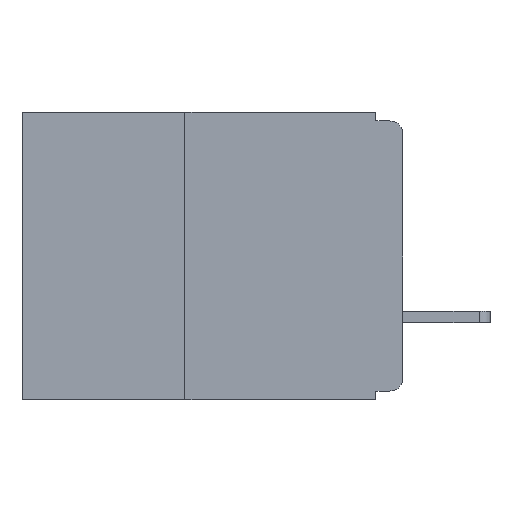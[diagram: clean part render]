
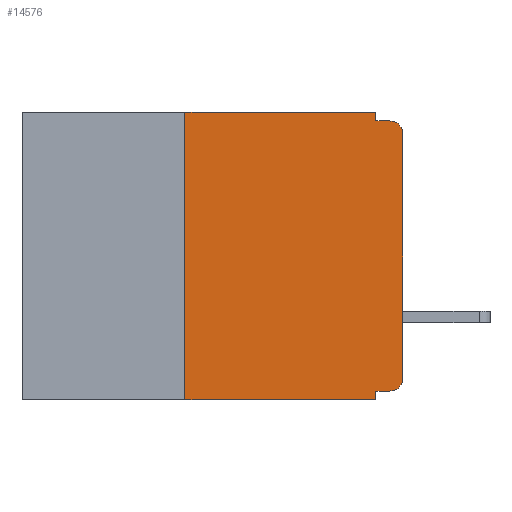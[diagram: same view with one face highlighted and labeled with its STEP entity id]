
A CAD part, left-side view. The second image highlights one B-rep face of the part: STEP entity #14576.
In plain terms, the highlighted planar face has unit normal (-1, 0, 0).
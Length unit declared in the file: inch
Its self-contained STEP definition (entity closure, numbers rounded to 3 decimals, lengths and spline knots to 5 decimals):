
#92 = CARTESIAN_POINT ( 'NONE',  ( 0., 0.437, 0. ) ) ;
#424 = DIRECTION ( 'NONE',  ( 0., -1., 0. ) ) ;
#1091 = VERTEX_POINT ( 'NONE', #3690 ) ;
#1225 = VECTOR ( 'NONE', #11261, 39.37008 ) ;
#1255 = CIRCLE ( 'NONE', #15630, 0.015 ) ;
#1487 = DIRECTION ( 'NONE',  ( 0., 0., -1. ) ) ;
#1725 = EDGE_CURVE ( 'NONE', #17184, #8489, #7365, .T. ) ;
#2604 = CARTESIAN_POINT ( 'NONE',  ( 0., 0.031, -0.32 ) ) ;
#2712 = LINE ( 'NONE', #20183, #19629 ) ;
#3062 = VERTEX_POINT ( 'NONE', #12607 ) ;
#3492 = LINE ( 'NONE', #15815, #20405 ) ;
#3570 = VECTOR ( 'NONE', #16879, 39.37008 ) ;
#3690 = CARTESIAN_POINT ( 'NONE',  ( 0., 0., -0.305 ) ) ;
#3854 = VERTEX_POINT ( 'NONE', #2604 ) ;
#4379 = LINE ( 'NONE', #15457, #8277 ) ;
#4683 = EDGE_CURVE ( 'NONE', #3854, #17141, #18455, .T. ) ;
#4888 = FACE_OUTER_BOUND ( 'NONE', #12258, .T. ) ;
#4970 = CARTESIAN_POINT ( 'NONE',  ( 0., 0.015, -0.305 ) ) ;
#5569 = DIRECTION ( 'NONE',  ( 0., 0., -1. ) ) ;
#5572 = CARTESIAN_POINT ( 'NONE',  ( 0., 0.031, -0.33 ) ) ;
#5885 = ORIENTED_EDGE ( 'NONE', *, *, #14229, .F. ) ;
#6247 = CARTESIAN_POINT ( 'NONE',  ( 0., 0.031, 0. ) ) ;
#6640 = DIRECTION ( 'NONE',  ( 0., 0., -1. ) ) ;
#6852 = VECTOR ( 'NONE', #18225, 39.37008 ) ;
#7365 = LINE ( 'NONE', #92, #6852 ) ;
#7405 = EDGE_CURVE ( 'NONE', #17925, #1091, #1255, .T. ) ;
#8218 = CARTESIAN_POINT ( 'NONE',  ( 0., 0.25, 0. ) ) ;
#8277 = VECTOR ( 'NONE', #17055, 39.37008 ) ;
#8302 = VERTEX_POINT ( 'NONE', #16017 ) ;
#8489 = VERTEX_POINT ( 'NONE', #21408 ) ;
#8665 = CARTESIAN_POINT ( 'NONE',  ( 0., 0.015, -0.025 ) ) ;
#9209 = EDGE_CURVE ( 'NONE', #3062, #17184, #16672, .T. ) ;
#9489 = ORIENTED_EDGE ( 'NONE', *, *, #1725, .F. ) ;
#9824 = VECTOR ( 'NONE', #5569, 39.37008 ) ;
#10168 = CIRCLE ( 'NONE', #20883, 0.015 ) ;
#10354 = DIRECTION ( 'NONE',  ( 0., 0., -1. ) ) ;
#10603 = ORIENTED_EDGE ( 'NONE', *, *, #4683, .F. ) ;
#10755 = CARTESIAN_POINT ( 'NONE',  ( 0., 0.031, -0.01 ) ) ;
#10818 = VECTOR ( 'NONE', #18946, 39.37008 ) ;
#10956 = ORIENTED_EDGE ( 'NONE', *, *, #20206, .T. ) ;
#10995 = DIRECTION ( 'NONE',  ( 0., 0., 1. ) ) ;
#11155 = ORIENTED_EDGE ( 'NONE', *, *, #11490, .T. ) ;
#11175 = ORIENTED_EDGE ( 'NONE', *, *, #7405, .T. ) ;
#11261 = DIRECTION ( 'NONE',  ( 0., 0., -1. ) ) ;
#11490 = EDGE_CURVE ( 'NONE', #1091, #8302, #3492, .T. ) ;
#11495 = DIRECTION ( 'NONE',  ( 1., 0., 0. ) ) ;
#12258 = EDGE_LOOP ( 'NONE', ( #11155, #10956, #13366, #14805, #9489, #21401, #19402, #10603, #5885, #11175 ) ) ;
#12607 = CARTESIAN_POINT ( 'NONE',  ( 0., 0.25, -0.33 ) ) ;
#13366 = ORIENTED_EDGE ( 'NONE', *, *, #16422, .F. ) ;
#13473 = LINE ( 'NONE', #6247, #1225 ) ;
#14229 = EDGE_CURVE ( 'NONE', #17925, #3854, #4379, .T. ) ;
#14576 = ADVANCED_FACE ( 'NONE', ( #4888 ), #21187, .F. ) ;
#14805 = ORIENTED_EDGE ( 'NONE', *, *, #21055, .F. ) ;
#14976 = VERTEX_POINT ( 'NONE', #10755 ) ;
#15276 = CARTESIAN_POINT ( 'NONE',  ( 0., 0.25, -0.33 ) ) ;
#15457 = CARTESIAN_POINT ( 'NONE',  ( 0., 0., -0.32 ) ) ;
#15630 = AXIS2_PLACEMENT_3D ( 'NONE', #4970, #16441, #6640 ) ;
#15773 = CARTESIAN_POINT ( 'NONE',  ( 0., 0., -0.01 ) ) ;
#15815 = CARTESIAN_POINT ( 'NONE',  ( 0., 0., 0. ) ) ;
#16017 = CARTESIAN_POINT ( 'NONE',  ( 0., 0., -0.025 ) ) ;
#16158 = VERTEX_POINT ( 'NONE', #18904 ) ;
#16392 = AXIS2_PLACEMENT_3D ( 'NONE', #17905, #11495, #1487 ) ;
#16422 = EDGE_CURVE ( 'NONE', #14976, #16158, #19419, .T. ) ;
#16441 = DIRECTION ( 'NONE',  ( -1., 0., 0. ) ) ;
#16672 = LINE ( 'NONE', #15276, #3570 ) ;
#16879 = DIRECTION ( 'NONE',  ( 0., 0., 1. ) ) ;
#17055 = DIRECTION ( 'NONE',  ( 0., 1., 0. ) ) ;
#17141 = VERTEX_POINT ( 'NONE', #21129 ) ;
#17184 = VERTEX_POINT ( 'NONE', #8218 ) ;
#17391 = EDGE_CURVE ( 'NONE', #3062, #17141, #2712, .T. ) ;
#17905 = CARTESIAN_POINT ( 'NONE',  ( 0., 0.437, 0. ) ) ;
#17925 = VERTEX_POINT ( 'NONE', #18160 ) ;
#18160 = CARTESIAN_POINT ( 'NONE',  ( 0., 0.015, -0.32 ) ) ;
#18225 = DIRECTION ( 'NONE',  ( 0., -1., 0. ) ) ;
#18455 = LINE ( 'NONE', #5572, #9824 ) ;
#18904 = CARTESIAN_POINT ( 'NONE',  ( 0., 0.015, -0.01 ) ) ;
#18946 = DIRECTION ( 'NONE',  ( 0., -1., 0. ) ) ;
#19402 = ORIENTED_EDGE ( 'NONE', *, *, #17391, .T. ) ;
#19419 = LINE ( 'NONE', #15773, #10818 ) ;
#19629 = VECTOR ( 'NONE', #424, 39.37008 ) ;
#20064 = DIRECTION ( 'NONE',  ( -1., 0., 0. ) ) ;
#20183 = CARTESIAN_POINT ( 'NONE',  ( 0., 0.437, -0.33 ) ) ;
#20206 = EDGE_CURVE ( 'NONE', #8302, #16158, #10168, .T. ) ;
#20405 = VECTOR ( 'NONE', #10995, 39.37008 ) ;
#20883 = AXIS2_PLACEMENT_3D ( 'NONE', #8665, #20064, #10354 ) ;
#21055 = EDGE_CURVE ( 'NONE', #8489, #14976, #13473, .T. ) ;
#21129 = CARTESIAN_POINT ( 'NONE',  ( 0., 0.031, -0.33 ) ) ;
#21187 = PLANE ( 'NONE',  #16392 ) ;
#21401 = ORIENTED_EDGE ( 'NONE', *, *, #9209, .F. ) ;
#21408 = CARTESIAN_POINT ( 'NONE',  ( 0., 0.031, 0. ) ) ;
